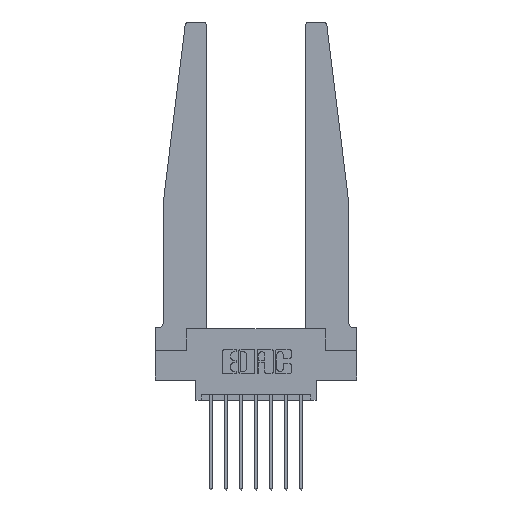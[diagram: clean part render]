
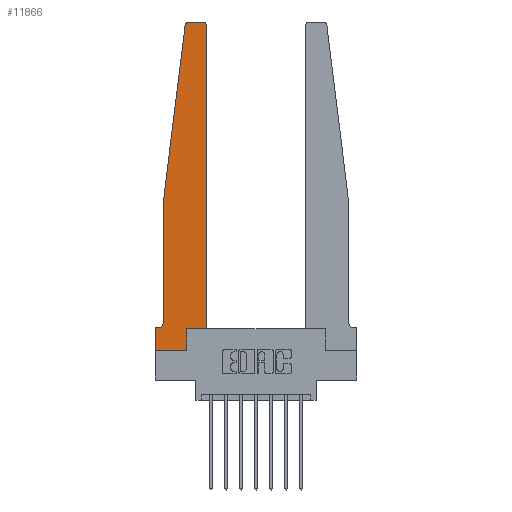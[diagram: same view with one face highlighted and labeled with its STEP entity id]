
A CAD part, top view. The second image highlights one B-rep face of the part: STEP entity #11866.
In plain terms, the highlighted planar face has unit normal (0, 0, 1).
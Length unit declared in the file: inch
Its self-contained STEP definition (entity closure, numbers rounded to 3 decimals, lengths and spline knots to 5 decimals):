
#236 = VECTOR ( 'NONE', #11615, 39.37008 ) ;
#596 = EDGE_LOOP ( 'NONE', ( #9382, #9763, #10870, #1251, #3924, #3811, #3014, #8805, #8489, #2357, #7504, #2847 ) ) ;
#812 = EDGE_CURVE ( 'NONE', #9677, #12131, #7393, .T. ) ;
#1088 = VERTEX_POINT ( 'NONE', #5203 ) ;
#1251 = ORIENTED_EDGE ( 'NONE', *, *, #12478, .T. ) ;
#1398 = VERTEX_POINT ( 'NONE', #5841 ) ;
#1486 = CIRCLE ( 'NONE', #3324, 0.03 ) ;
#1558 = CARTESIAN_POINT ( 'NONE',  ( 0.425, 0.18, 0.37 ) ) ;
#1584 = VERTEX_POINT ( 'NONE', #9410 ) ;
#1721 = CARTESIAN_POINT ( 'NONE',  ( 0.015, 0.1875, 0.37 ) ) ;
#1775 = AXIS2_PLACEMENT_3D ( 'NONE', #12920, #8670, #2035 ) ;
#1903 = EDGE_CURVE ( 'NONE', #1398, #5436, #8312, .T. ) ;
#1929 = CARTESIAN_POINT ( 'NONE',  ( 0.065, 0.1875, 0.37 ) ) ;
#1959 = VECTOR ( 'NONE', #4989, 39.37008 ) ;
#1986 = PLANE ( 'NONE',  #1775 ) ;
#2002 = CARTESIAN_POINT ( 'NONE',  ( 0., 0., 0.37 ) ) ;
#2035 = DIRECTION ( 'NONE',  ( 1., 0., 0. ) ) ;
#2055 = EDGE_CURVE ( 'NONE', #12131, #2850, #3229, .T. ) ;
#2340 = CARTESIAN_POINT ( 'NONE',  ( 0., 0.1875, 0.37 ) ) ;
#2357 = ORIENTED_EDGE ( 'NONE', *, *, #9594, .T. ) ;
#2536 = CARTESIAN_POINT ( 'NONE',  ( 0.27653, 2.72, 0.37 ) ) ;
#2847 = ORIENTED_EDGE ( 'NONE', *, *, #8351, .T. ) ;
#2850 = VERTEX_POINT ( 'NONE', #14045 ) ;
#2904 = AXIS2_PLACEMENT_3D ( 'NONE', #10287, #3714, #11372 ) ;
#2940 = VECTOR ( 'NONE', #8847, 39.37008 ) ;
#3014 = ORIENTED_EDGE ( 'NONE', *, *, #13708, .T. ) ;
#3229 = LINE ( 'NONE', #10523, #236 ) ;
#3324 = AXIS2_PLACEMENT_3D ( 'NONE', #3988, #11644, #5116 ) ;
#3596 = AXIS2_PLACEMENT_3D ( 'NONE', #2536, #10252, #3669 ) ;
#3669 = DIRECTION ( 'NONE',  ( 1., 0., 0. ) ) ;
#3701 = VECTOR ( 'NONE', #14188, 39.37008 ) ;
#3711 = DIRECTION ( 'NONE',  ( -0.122, -0.992, 0. ) ) ;
#3714 = DIRECTION ( 'NONE',  ( 0., 0., -1. ) ) ;
#3811 = ORIENTED_EDGE ( 'NONE', *, *, #7765, .T. ) ;
#3924 = ORIENTED_EDGE ( 'NONE', *, *, #5212, .T. ) ;
#3988 = CARTESIAN_POINT ( 'NONE',  ( 0.395, 2.72, 0.37 ) ) ;
#4037 = CARTESIAN_POINT ( 'NONE',  ( 0.24675, 2.72367, 0.37 ) ) ;
#4325 = CARTESIAN_POINT ( 'NONE',  ( 0., 0., 0.37 ) ) ;
#4333 = VECTOR ( 'NONE', #3711, 39.37008 ) ;
#4412 = EDGE_CURVE ( 'NONE', #5268, #1088, #4934, .T. ) ;
#4803 = EDGE_CURVE ( 'NONE', #8814, #1398, #12418, .T. ) ;
#4934 = LINE ( 'NONE', #10435, #1959 ) ;
#4989 = DIRECTION ( 'NONE',  ( 0., 1., 0. ) ) ;
#5031 = VECTOR ( 'NONE', #5447, 39.37008 ) ;
#5116 = DIRECTION ( 'NONE',  ( 1., 0., 0. ) ) ;
#5203 = CARTESIAN_POINT ( 'NONE',  ( 0.425, 2.72, 0.37 ) ) ;
#5212 = EDGE_CURVE ( 'NONE', #1584, #6368, #7705, .T. ) ;
#5268 = VERTEX_POINT ( 'NONE', #1558 ) ;
#5436 = VERTEX_POINT ( 'NONE', #4037 ) ;
#5447 = DIRECTION ( 'NONE',  ( 0., -1., 0. ) ) ;
#5461 = VECTOR ( 'NONE', #13818, 39.37008 ) ;
#5477 = VERTEX_POINT ( 'NONE', #9609 ) ;
#5754 = CARTESIAN_POINT ( 'NONE',  ( 0., 0., 0.37 ) ) ;
#5841 = CARTESIAN_POINT ( 'NONE',  ( 0.27653, 2.75, 0.37 ) ) ;
#5937 = LINE ( 'NONE', #1929, #14172 ) ;
#6368 = VERTEX_POINT ( 'NONE', #1721 ) ;
#6649 = CARTESIAN_POINT ( 'NONE',  ( 0.065, 1.25, 0.37 ) ) ;
#7121 = CARTESIAN_POINT ( 'NONE',  ( 0.395, 2.75, 0.37 ) ) ;
#7393 = LINE ( 'NONE', #5754, #10239 ) ;
#7504 = ORIENTED_EDGE ( 'NONE', *, *, #4412, .T. ) ;
#7697 = FACE_OUTER_BOUND ( 'NONE', #596, .T. ) ;
#7705 = CIRCLE ( 'NONE', #2904, 0.05 ) ;
#7765 = EDGE_CURVE ( 'NONE', #6368, #9276, #5937, .T. ) ;
#8312 = CIRCLE ( 'NONE', #3596, 0.03 ) ;
#8351 = EDGE_CURVE ( 'NONE', #1088, #8814, #1486, .T. ) ;
#8489 = ORIENTED_EDGE ( 'NONE', *, *, #2055, .T. ) ;
#8670 = DIRECTION ( 'NONE',  ( 0., 0., 1. ) ) ;
#8805 = ORIENTED_EDGE ( 'NONE', *, *, #812, .T. ) ;
#8814 = VERTEX_POINT ( 'NONE', #7121 ) ;
#8845 = LINE ( 'NONE', #6649, #2940 ) ;
#8847 = DIRECTION ( 'NONE',  ( 0., -1., 0. ) ) ;
#9276 = VERTEX_POINT ( 'NONE', #2340 ) ;
#9382 = ORIENTED_EDGE ( 'NONE', *, *, #4803, .T. ) ;
#9410 = CARTESIAN_POINT ( 'NONE',  ( 0.065, 0.2375, 0.37 ) ) ;
#9594 = EDGE_CURVE ( 'NONE', #2850, #5268, #11601, .T. ) ;
#9609 = CARTESIAN_POINT ( 'NONE',  ( 0.065, 1.25, 0.37 ) ) ;
#9677 = VERTEX_POINT ( 'NONE', #2002 ) ;
#9763 = ORIENTED_EDGE ( 'NONE', *, *, #1903, .T. ) ;
#10239 = VECTOR ( 'NONE', #12209, 39.37008 ) ;
#10252 = DIRECTION ( 'NONE',  ( 0., 0., 1. ) ) ;
#10287 = CARTESIAN_POINT ( 'NONE',  ( 0.015, 0.2375, 0.37 ) ) ;
#10435 = CARTESIAN_POINT ( 'NONE',  ( 0.425, 0.18, 0.37 ) ) ;
#10523 = CARTESIAN_POINT ( 'NONE',  ( 0.2605, 0.18, 0.37 ) ) ;
#10870 = ORIENTED_EDGE ( 'NONE', *, *, #13341, .T. ) ;
#11368 = CARTESIAN_POINT ( 'NONE',  ( 0.065, 1.25, 0.37 ) ) ;
#11372 = DIRECTION ( 'NONE',  ( -1., 0., 0. ) ) ;
#11519 = LINE ( 'NONE', #4325, #5031 ) ;
#11601 = LINE ( 'NONE', #12763, #5461 ) ;
#11615 = DIRECTION ( 'NONE',  ( 0., 1., 0. ) ) ;
#11644 = DIRECTION ( 'NONE',  ( 0., 0., 1. ) ) ;
#11866 = ADVANCED_FACE ( 'NONE', ( #7697 ), #1986, .T. ) ;
#12131 = VERTEX_POINT ( 'NONE', #12336 ) ;
#12209 = DIRECTION ( 'NONE',  ( 1., 0., 0. ) ) ;
#12336 = CARTESIAN_POINT ( 'NONE',  ( 0.2605, 0., 0.37 ) ) ;
#12418 = LINE ( 'NONE', #13120, #3701 ) ;
#12478 = EDGE_CURVE ( 'NONE', #5477, #1584, #8845, .T. ) ;
#12763 = CARTESIAN_POINT ( 'NONE',  ( 0.425, 0.18, 0.37 ) ) ;
#12920 = CARTESIAN_POINT ( 'NONE',  ( 0., 0.1875, 0.37 ) ) ;
#13001 = LINE ( 'NONE', #11368, #4333 ) ;
#13120 = CARTESIAN_POINT ( 'NONE',  ( 0.25, 2.75, 0.37 ) ) ;
#13341 = EDGE_CURVE ( 'NONE', #5436, #5477, #13001, .T. ) ;
#13708 = EDGE_CURVE ( 'NONE', #9276, #9677, #11519, .T. ) ;
#13818 = DIRECTION ( 'NONE',  ( 1., 0., 0. ) ) ;
#13891 = DIRECTION ( 'NONE',  ( -1., 0., 0. ) ) ;
#14045 = CARTESIAN_POINT ( 'NONE',  ( 0.2605, 0.18, 0.37 ) ) ;
#14172 = VECTOR ( 'NONE', #13891, 39.37008 ) ;
#14188 = DIRECTION ( 'NONE',  ( -1., 0., 0. ) ) ;
